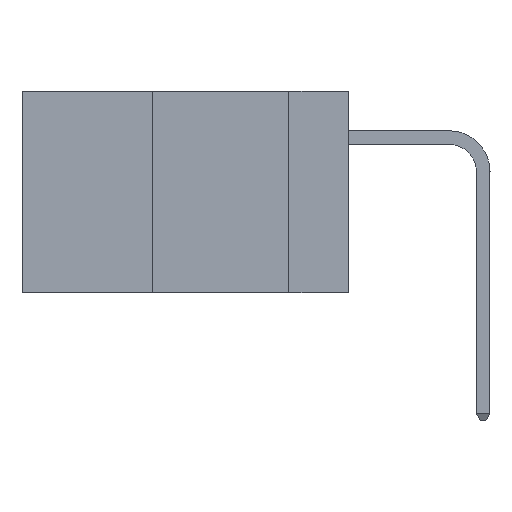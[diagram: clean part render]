
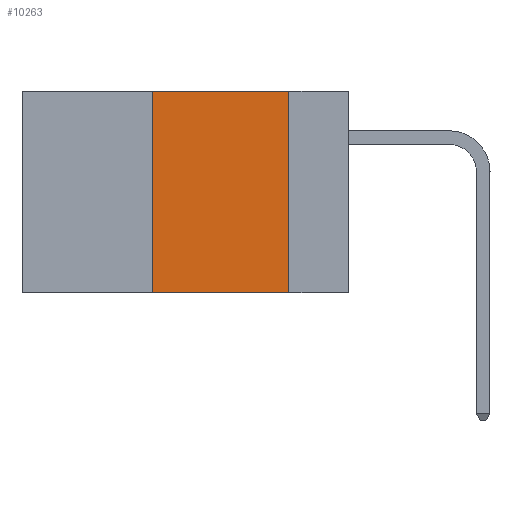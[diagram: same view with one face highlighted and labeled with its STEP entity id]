
A CAD part, left-side view. The second image highlights one B-rep face of the part: STEP entity #10263.
In plain terms, the highlighted planar face has unit normal (-1, 0, 0).
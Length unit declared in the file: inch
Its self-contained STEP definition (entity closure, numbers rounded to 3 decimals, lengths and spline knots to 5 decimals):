
#112 = EDGE_LOOP ( 'NONE', ( #9095, #4043, #20889, #16838 ) ) ;
#771 = DIRECTION ( 'NONE',  ( 0., -1., 0. ) ) ;
#850 = VECTOR ( 'NONE', #15028, 39.37008 ) ;
#1457 = LINE ( 'NONE', #18826, #850 ) ;
#2028 = VERTEX_POINT ( 'NONE', #4854 ) ;
#2960 = EDGE_CURVE ( 'NONE', #11984, #12255, #1457, .T. ) ;
#3248 = CARTESIAN_POINT ( 'NONE',  ( 0., 0.11, -0.37 ) ) ;
#3279 = AXIS2_PLACEMENT_3D ( 'NONE', #14434, #7220, #13764 ) ;
#4043 = ORIENTED_EDGE ( 'NONE', *, *, #7495, .F. ) ;
#4819 = CARTESIAN_POINT ( 'NONE',  ( 0., 0.6, -0.37 ) ) ;
#4854 = CARTESIAN_POINT ( 'NONE',  ( 0., 0.36, 0. ) ) ;
#7006 = CARTESIAN_POINT ( 'NONE',  ( 0., 0.36, -0.37 ) ) ;
#7220 = DIRECTION ( 'NONE',  ( 1., 0., 0. ) ) ;
#7495 = EDGE_CURVE ( 'NONE', #2028, #11984, #17514, .T. ) ;
#8021 = FACE_OUTER_BOUND ( 'NONE', #112, .T. ) ;
#8196 = CARTESIAN_POINT ( 'NONE',  ( 0., 0.6, 0. ) ) ;
#8398 = VECTOR ( 'NONE', #771, 39.37008 ) ;
#8518 = VECTOR ( 'NONE', #11277, 39.37008 ) ;
#9095 = ORIENTED_EDGE ( 'NONE', *, *, #2960, .F. ) ;
#10263 = ADVANCED_FACE ( 'NONE', ( #8021 ), #16280, .F. ) ;
#11277 = DIRECTION ( 'NONE',  ( 0., 0., 1. ) ) ;
#11984 = VERTEX_POINT ( 'NONE', #16694 ) ;
#12255 = VERTEX_POINT ( 'NONE', #3248 ) ;
#13764 = DIRECTION ( 'NONE',  ( 0., 0., -1. ) ) ;
#13935 = DIRECTION ( 'NONE',  ( 0., -1., 0. ) ) ;
#14434 = CARTESIAN_POINT ( 'NONE',  ( 0., 0.6, 0. ) ) ;
#15028 = DIRECTION ( 'NONE',  ( 0., 0., -1. ) ) ;
#16280 = PLANE ( 'NONE',  #3279 ) ;
#16694 = CARTESIAN_POINT ( 'NONE',  ( 0., 0.11, 0. ) ) ;
#16838 = ORIENTED_EDGE ( 'NONE', *, *, #19045, .T. ) ;
#17260 = EDGE_CURVE ( 'NONE', #22247, #2028, #18225, .T. ) ;
#17514 = LINE ( 'NONE', #8196, #8398 ) ;
#18225 = LINE ( 'NONE', #20340, #8518 ) ;
#18826 = CARTESIAN_POINT ( 'NONE',  ( 0., 0.11, 0. ) ) ;
#19045 = EDGE_CURVE ( 'NONE', #22247, #12255, #21254, .T. ) ;
#20340 = CARTESIAN_POINT ( 'NONE',  ( 0., 0.36, 0. ) ) ;
#20692 = VECTOR ( 'NONE', #13935, 39.37008 ) ;
#20889 = ORIENTED_EDGE ( 'NONE', *, *, #17260, .F. ) ;
#21254 = LINE ( 'NONE', #4819, #20692 ) ;
#22247 = VERTEX_POINT ( 'NONE', #7006 ) ;
